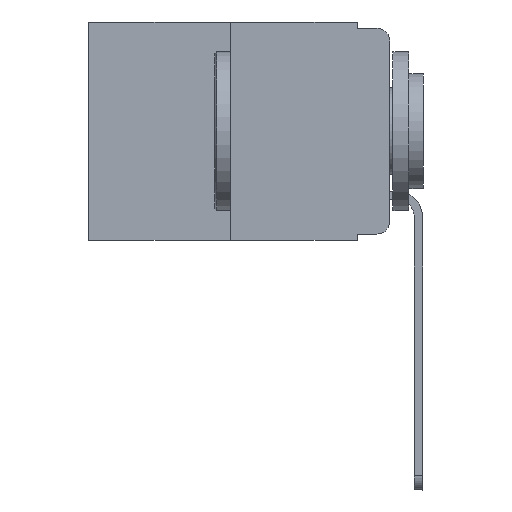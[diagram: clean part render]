
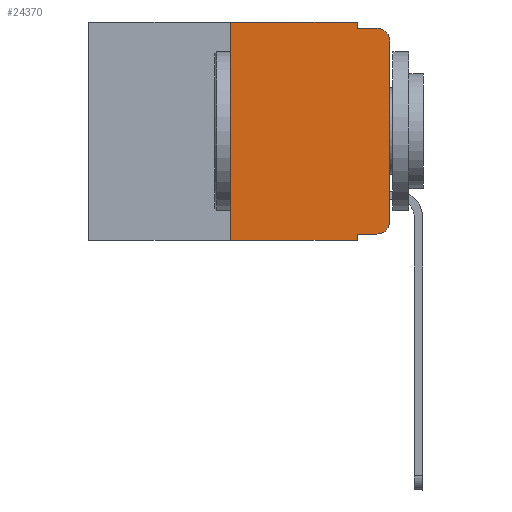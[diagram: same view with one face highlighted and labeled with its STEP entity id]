
A CAD part, left-side view. The second image highlights one B-rep face of the part: STEP entity #24370.
In plain terms, the highlighted planar face has unit normal (-1, 0, 0).
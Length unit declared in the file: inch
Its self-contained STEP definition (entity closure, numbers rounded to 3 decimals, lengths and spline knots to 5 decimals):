
#38 = EDGE_CURVE ( 'NONE', #17466, #14487, #5671, .T. ) ;
#283 = CARTESIAN_POINT ( 'NONE',  ( 0., 0.051, 0. ) ) ;
#387 = DIRECTION ( 'NONE',  ( 0., -1., 0. ) ) ;
#773 = VERTEX_POINT ( 'NONE', #22732 ) ;
#851 = VERTEX_POINT ( 'NONE', #13330 ) ;
#1181 = PLANE ( 'NONE',  #9035 ) ;
#1297 = EDGE_CURVE ( 'NONE', #14487, #22772, #1617, .T. ) ;
#1617 = CIRCLE ( 'NONE', #6527, 0.02 ) ;
#1927 = ORIENTED_EDGE ( 'NONE', *, *, #21313, .F. ) ;
#2206 = VECTOR ( 'NONE', #8336, 39.37008 ) ;
#2575 = EDGE_CURVE ( 'NONE', #18533, #3871, #17426, .T. ) ;
#3179 = EDGE_CURVE ( 'NONE', #22772, #8553, #21500, .T. ) ;
#3424 = CARTESIAN_POINT ( 'NONE',  ( 0., 0.25, -0.343 ) ) ;
#3612 = CARTESIAN_POINT ( 'NONE',  ( 0., 0.051, -0.01 ) ) ;
#3809 = ORIENTED_EDGE ( 'NONE', *, *, #5113, .F. ) ;
#3871 = VERTEX_POINT ( 'NONE', #20166 ) ;
#4711 = ORIENTED_EDGE ( 'NONE', *, *, #20944, .T. ) ;
#5113 = EDGE_CURVE ( 'NONE', #12673, #12384, #9255, .T. ) ;
#5407 = EDGE_CURVE ( 'NONE', #3871, #773, #22860, .T. ) ;
#5671 = LINE ( 'NONE', #15474, #10978 ) ;
#6527 = AXIS2_PLACEMENT_3D ( 'NONE', #19354, #22958, #25277 ) ;
#6829 = CARTESIAN_POINT ( 'NONE',  ( 0., 0.02, -0.333 ) ) ;
#7362 = DIRECTION ( 'NONE',  ( 0., 0., 1. ) ) ;
#7725 = DIRECTION ( 'NONE',  ( 0., 0., -1. ) ) ;
#8216 = ORIENTED_EDGE ( 'NONE', *, *, #38, .T. ) ;
#8336 = DIRECTION ( 'NONE',  ( 0., 0., 1. ) ) ;
#8553 = VERTEX_POINT ( 'NONE', #14366 ) ;
#8598 = DIRECTION ( 'NONE',  ( 0., 0., -1. ) ) ;
#8721 = CARTESIAN_POINT ( 'NONE',  ( 0., 0.02, -0.03 ) ) ;
#8974 = DIRECTION ( 'NONE',  ( -1., 0., 0. ) ) ;
#9009 = CARTESIAN_POINT ( 'NONE',  ( 0., 0.473, 0. ) ) ;
#9035 = AXIS2_PLACEMENT_3D ( 'NONE', #9009, #22807, #24742 ) ;
#9255 = LINE ( 'NONE', #3612, #11696 ) ;
#10408 = EDGE_CURVE ( 'NONE', #17466, #851, #21909, .T. ) ;
#10590 = ORIENTED_EDGE ( 'NONE', *, *, #1297, .T. ) ;
#10978 = VECTOR ( 'NONE', #23078, 39.37008 ) ;
#11440 = DIRECTION ( 'NONE',  ( 0., -1., 0. ) ) ;
#11696 = VECTOR ( 'NONE', #11440, 39.37008 ) ;
#12075 = CARTESIAN_POINT ( 'NONE',  ( 0., 0.473, 0. ) ) ;
#12150 = CARTESIAN_POINT ( 'NONE',  ( 0., 0.051, -0.01 ) ) ;
#12188 = VECTOR ( 'NONE', #14214, 39.37008 ) ;
#12322 = ORIENTED_EDGE ( 'NONE', *, *, #10408, .F. ) ;
#12384 = VERTEX_POINT ( 'NONE', #14160 ) ;
#12494 = EDGE_CURVE ( 'NONE', #8553, #12384, #17679, .T. ) ;
#12673 = VERTEX_POINT ( 'NONE', #12150 ) ;
#12928 = ORIENTED_EDGE ( 'NONE', *, *, #3179, .T. ) ;
#13330 = CARTESIAN_POINT ( 'NONE',  ( 0., 0.051, -0.343 ) ) ;
#14025 = LINE ( 'NONE', #15960, #18802 ) ;
#14160 = CARTESIAN_POINT ( 'NONE',  ( 0., 0.02, -0.01 ) ) ;
#14214 = DIRECTION ( 'NONE',  ( 0., -1., 0. ) ) ;
#14366 = CARTESIAN_POINT ( 'NONE',  ( 0., 0., -0.03 ) ) ;
#14487 = VERTEX_POINT ( 'NONE', #6829 ) ;
#14585 = ORIENTED_EDGE ( 'NONE', *, *, #12494, .T. ) ;
#14710 = FACE_OUTER_BOUND ( 'NONE', #15979, .T. ) ;
#15474 = CARTESIAN_POINT ( 'NONE',  ( 0., 0.051, -0.333 ) ) ;
#15960 = CARTESIAN_POINT ( 'NONE',  ( 0., 0.051, 0. ) ) ;
#15979 = EDGE_LOOP ( 'NONE', ( #12928, #14585, #3809, #1927, #23491, #17498, #4711, #12322, #8216, #10590 ) ) ;
#16407 = LINE ( 'NONE', #24137, #12188 ) ;
#17172 = CARTESIAN_POINT ( 'NONE',  ( 0., 0.25, 0. ) ) ;
#17426 = LINE ( 'NONE', #17172, #18612 ) ;
#17466 = VERTEX_POINT ( 'NONE', #20232 ) ;
#17498 = ORIENTED_EDGE ( 'NONE', *, *, #2575, .F. ) ;
#17679 = CIRCLE ( 'NONE', #24682, 0.02 ) ;
#18533 = VERTEX_POINT ( 'NONE', #3424 ) ;
#18612 = VECTOR ( 'NONE', #7362, 39.37008 ) ;
#18745 = VECTOR ( 'NONE', #387, 39.37008 ) ;
#18802 = VECTOR ( 'NONE', #21878, 39.37008 ) ;
#19301 = VECTOR ( 'NONE', #7725, 39.37008 ) ;
#19354 = CARTESIAN_POINT ( 'NONE',  ( 0., 0.02, -0.313 ) ) ;
#20166 = CARTESIAN_POINT ( 'NONE',  ( 0., 0.25, 0. ) ) ;
#20232 = CARTESIAN_POINT ( 'NONE',  ( 0., 0.051, -0.333 ) ) ;
#20944 = EDGE_CURVE ( 'NONE', #18533, #851, #16407, .T. ) ;
#21313 = EDGE_CURVE ( 'NONE', #773, #12673, #14025, .T. ) ;
#21500 = LINE ( 'NONE', #21632, #2206 ) ;
#21632 = CARTESIAN_POINT ( 'NONE',  ( 0., 0., 0. ) ) ;
#21878 = DIRECTION ( 'NONE',  ( 0., 0., -1. ) ) ;
#21909 = LINE ( 'NONE', #283, #19301 ) ;
#22676 = CARTESIAN_POINT ( 'NONE',  ( 0., 0., -0.313 ) ) ;
#22732 = CARTESIAN_POINT ( 'NONE',  ( 0., 0.051, 0. ) ) ;
#22772 = VERTEX_POINT ( 'NONE', #22676 ) ;
#22807 = DIRECTION ( 'NONE',  ( 1., 0., 0. ) ) ;
#22860 = LINE ( 'NONE', #12075, #18745 ) ;
#22958 = DIRECTION ( 'NONE',  ( -1., 0., 0. ) ) ;
#23078 = DIRECTION ( 'NONE',  ( 0., -1., 0. ) ) ;
#23491 = ORIENTED_EDGE ( 'NONE', *, *, #5407, .F. ) ;
#24137 = CARTESIAN_POINT ( 'NONE',  ( 0., 0.473, -0.343 ) ) ;
#24370 = ADVANCED_FACE ( 'NONE', ( #14710 ), #1181, .F. ) ;
#24682 = AXIS2_PLACEMENT_3D ( 'NONE', #8721, #8974, #8598 ) ;
#24742 = DIRECTION ( 'NONE',  ( 0., 0., -1. ) ) ;
#25277 = DIRECTION ( 'NONE',  ( 0., 0., -1. ) ) ;
